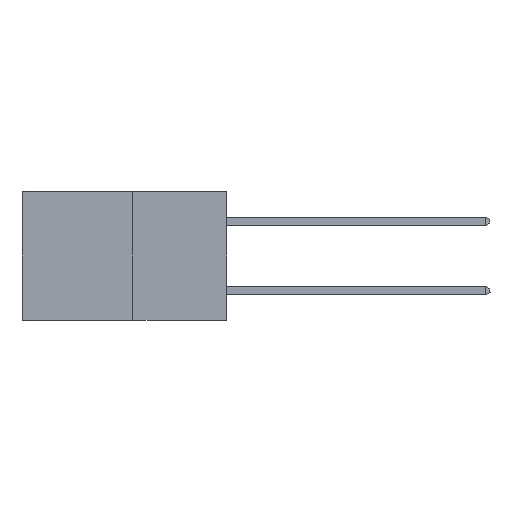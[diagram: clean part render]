
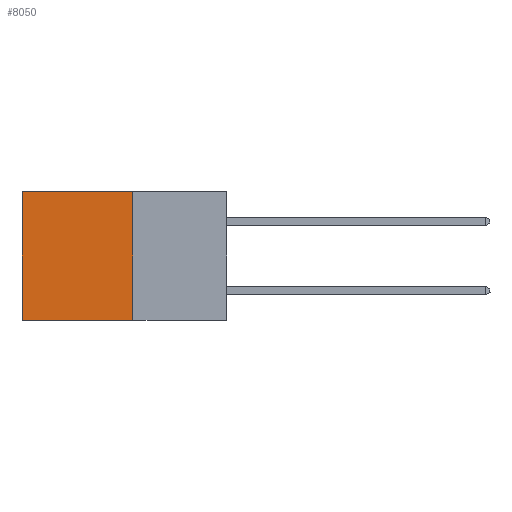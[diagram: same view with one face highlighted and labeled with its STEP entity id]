
A CAD part, left-side view. The second image highlights one B-rep face of the part: STEP entity #8050.
In plain terms, the highlighted planar face has unit normal (-1, 0, 0).
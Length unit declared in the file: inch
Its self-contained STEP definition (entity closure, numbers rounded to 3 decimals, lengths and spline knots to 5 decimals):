
#558 = PLANE ( 'NONE',  #14211 ) ;
#836 = EDGE_CURVE ( 'NONE', #12980, #5905, #2632, .T. ) ;
#977 = ORIENTED_EDGE ( 'NONE', *, *, #5427, .T. ) ;
#1205 = EDGE_CURVE ( 'NONE', #13506, #5905, #9993, .T. ) ;
#1254 = CARTESIAN_POINT ( 'NONE',  ( 0.277, 0.59, -0.37 ) ) ;
#1368 = VECTOR ( 'NONE', #8589, 39.37008 ) ;
#1748 = CARTESIAN_POINT ( 'NONE',  ( 0.277, 0.59, 0. ) ) ;
#1914 = CARTESIAN_POINT ( 'NONE',  ( 0.277, 0.27, -0.37 ) ) ;
#2632 = LINE ( 'NONE', #9599, #11174 ) ;
#3147 = VECTOR ( 'NONE', #12976, 39.37008 ) ;
#3459 = CARTESIAN_POINT ( 'NONE',  ( 0.277, 0.27, 0. ) ) ;
#3520 = LINE ( 'NONE', #1914, #3147 ) ;
#3967 = DIRECTION ( 'NONE',  ( 1., 0., 0. ) ) ;
#5143 = CARTESIAN_POINT ( 'NONE',  ( 0.277, 0.27, 0. ) ) ;
#5413 = DIRECTION ( 'NONE',  ( 0., 1., 0. ) ) ;
#5427 = EDGE_CURVE ( 'NONE', #9601, #12980, #9729, .T. ) ;
#5824 = ORIENTED_EDGE ( 'NONE', *, *, #1205, .F. ) ;
#5839 = ORIENTED_EDGE ( 'NONE', *, *, #11394, .F. ) ;
#5905 = VERTEX_POINT ( 'NONE', #1254 ) ;
#6759 = VECTOR ( 'NONE', #5413, 39.37008 ) ;
#6990 = EDGE_LOOP ( 'NONE', ( #8206, #5824, #5839, #977 ) ) ;
#8050 = ADVANCED_FACE ( 'NONE', ( #11921 ), #558, .F. ) ;
#8132 = DIRECTION ( 'NONE',  ( 0., 0., -1. ) ) ;
#8206 = ORIENTED_EDGE ( 'NONE', *, *, #836, .T. ) ;
#8589 = DIRECTION ( 'NONE',  ( 0., 1., 0. ) ) ;
#8765 = CARTESIAN_POINT ( 'NONE',  ( 0.277, 0.27, -0.37 ) ) ;
#9599 = CARTESIAN_POINT ( 'NONE',  ( 0.277, 0.59, -0.37 ) ) ;
#9601 = VERTEX_POINT ( 'NONE', #3459 ) ;
#9729 = LINE ( 'NONE', #5143, #6759 ) ;
#9993 = LINE ( 'NONE', #8765, #1368 ) ;
#10584 = CARTESIAN_POINT ( 'NONE',  ( 0.277, 0.27, -0.37 ) ) ;
#10670 = CARTESIAN_POINT ( 'NONE',  ( 0.277, 0.27, -0.37 ) ) ;
#11174 = VECTOR ( 'NONE', #8132, 39.37008 ) ;
#11394 = EDGE_CURVE ( 'NONE', #9601, #13506, #3520, .T. ) ;
#11710 = DIRECTION ( 'NONE',  ( 0., 0., -1. ) ) ;
#11921 = FACE_OUTER_BOUND ( 'NONE', #6990, .T. ) ;
#12976 = DIRECTION ( 'NONE',  ( 0., 0., -1. ) ) ;
#12980 = VERTEX_POINT ( 'NONE', #1748 ) ;
#13506 = VERTEX_POINT ( 'NONE', #10584 ) ;
#14211 = AXIS2_PLACEMENT_3D ( 'NONE', #10670, #3967, #11710 ) ;
